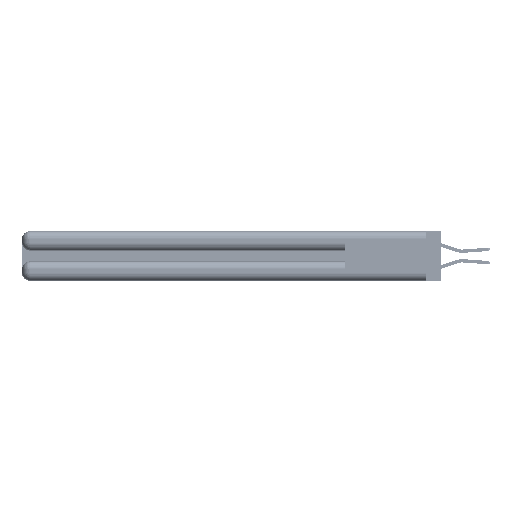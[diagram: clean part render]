
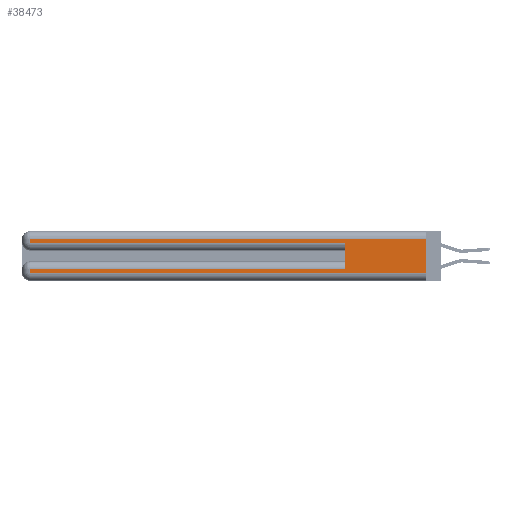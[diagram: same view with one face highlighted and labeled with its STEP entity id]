
A CAD part, left-side view. The second image highlights one B-rep face of the part: STEP entity #38473.
In plain terms, the highlighted planar face has unit normal (-1, 0, 0).
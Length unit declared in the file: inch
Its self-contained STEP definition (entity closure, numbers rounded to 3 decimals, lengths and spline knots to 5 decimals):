
#890 = CARTESIAN_POINT ( 'NONE',  ( 0., 2.94, 0.37 ) ) ;
#932 = VERTEX_POINT ( 'NONE', #32620 ) ;
#1877 = EDGE_CURVE ( 'NONE', #35243, #2897, #27796, .T. ) ;
#2897 = VERTEX_POINT ( 'NONE', #12723 ) ;
#3197 = ORIENTED_EDGE ( 'NONE', *, *, #33823, .F. ) ;
#3371 = CARTESIAN_POINT ( 'NONE',  ( 0., 0.6, 0.285 ) ) ;
#3842 = AXIS2_PLACEMENT_3D ( 'NONE', #46425, #28708, #24818 ) ;
#5562 = LINE ( 'NONE', #17791, #46593 ) ;
#5864 = DIRECTION ( 'NONE',  ( 0., -1., 0. ) ) ;
#5989 = CARTESIAN_POINT ( 'NONE',  ( 0., 2.94, 0.37 ) ) ;
#6622 = CARTESIAN_POINT ( 'NONE',  ( 0., 0., 0.06 ) ) ;
#7328 = DIRECTION ( 'NONE',  ( 0., 0., -1. ) ) ;
#9980 = VECTOR ( 'NONE', #13212, 39.37008 ) ;
#10544 = ORIENTED_EDGE ( 'NONE', *, *, #23265, .T. ) ;
#11126 = VECTOR ( 'NONE', #21945, 39.37008 ) ;
#11257 = ORIENTED_EDGE ( 'NONE', *, *, #32932, .T. ) ;
#11931 = ORIENTED_EDGE ( 'NONE', *, *, #38684, .T. ) ;
#12723 = CARTESIAN_POINT ( 'NONE',  ( 0., 0., 0.06 ) ) ;
#13212 = DIRECTION ( 'NONE',  ( 0., 0., -1. ) ) ;
#14539 = LINE ( 'NONE', #35554, #11126 ) ;
#15674 = VERTEX_POINT ( 'NONE', #33272 ) ;
#16194 = VERTEX_POINT ( 'NONE', #19778 ) ;
#17791 = CARTESIAN_POINT ( 'NONE',  ( 0., 0., 0.285 ) ) ;
#19778 = CARTESIAN_POINT ( 'NONE',  ( 0., 2.94, 0.085 ) ) ;
#20810 = ORIENTED_EDGE ( 'NONE', *, *, #1877, .F. ) ;
#21945 = DIRECTION ( 'NONE',  ( 0., 1., 0. ) ) ;
#21985 = CARTESIAN_POINT ( 'NONE',  ( 0., 0., 0.37 ) ) ;
#23182 = VECTOR ( 'NONE', #54399, 39.37008 ) ;
#23265 = EDGE_CURVE ( 'NONE', #15674, #24931, #47093, .T. ) ;
#23719 = VECTOR ( 'NONE', #32112, 39.37008 ) ;
#24041 = LINE ( 'NONE', #6622, #41199 ) ;
#24818 = DIRECTION ( 'NONE',  ( 0., 0., -1. ) ) ;
#24931 = VERTEX_POINT ( 'NONE', #40287 ) ;
#25296 = EDGE_LOOP ( 'NONE', ( #20810, #11931, #10544, #47785, #3197, #11257, #41874, #27517 ) ) ;
#27302 = DIRECTION ( 'NONE',  ( 0., 0., -1. ) ) ;
#27517 = ORIENTED_EDGE ( 'NONE', *, *, #31143, .T. ) ;
#27543 = EDGE_CURVE ( 'NONE', #16194, #932, #53523, .T. ) ;
#27796 = LINE ( 'NONE', #21985, #9980 ) ;
#28708 = DIRECTION ( 'NONE',  ( 1., 0., 0. ) ) ;
#30741 = LINE ( 'NONE', #32299, #23182 ) ;
#31143 = EDGE_CURVE ( 'NONE', #932, #2897, #24041, .T. ) ;
#32112 = DIRECTION ( 'NONE',  ( 0., 0., 1. ) ) ;
#32299 = CARTESIAN_POINT ( 'NONE',  ( 0., 0., 0.085 ) ) ;
#32620 = CARTESIAN_POINT ( 'NONE',  ( 0., 2.94, 0.06 ) ) ;
#32932 = EDGE_CURVE ( 'NONE', #41342, #16194, #30741, .T. ) ;
#33272 = CARTESIAN_POINT ( 'NONE',  ( 0., 2.94, 0.31 ) ) ;
#33823 = EDGE_CURVE ( 'NONE', #41342, #43719, #39517, .T. ) ;
#34860 = VECTOR ( 'NONE', #27302, 39.37008 ) ;
#35243 = VERTEX_POINT ( 'NONE', #54662 ) ;
#35554 = CARTESIAN_POINT ( 'NONE',  ( 0., 0., 0.31 ) ) ;
#38473 = ADVANCED_FACE ( 'NONE', ( #53553 ), #55399, .F. ) ;
#38684 = EDGE_CURVE ( 'NONE', #35243, #15674, #14539, .T. ) ;
#39517 = LINE ( 'NONE', #49441, #23719 ) ;
#40287 = CARTESIAN_POINT ( 'NONE',  ( 0., 2.94, 0.285 ) ) ;
#41199 = VECTOR ( 'NONE', #5864, 39.37008 ) ;
#41342 = VERTEX_POINT ( 'NONE', #48797 ) ;
#41874 = ORIENTED_EDGE ( 'NONE', *, *, #27543, .T. ) ;
#43719 = VERTEX_POINT ( 'NONE', #3371 ) ;
#46425 = CARTESIAN_POINT ( 'NONE',  ( 0., 0., 0.37 ) ) ;
#46593 = VECTOR ( 'NONE', #52581, 39.37008 ) ;
#46753 = EDGE_CURVE ( 'NONE', #24931, #43719, #5562, .T. ) ;
#47093 = LINE ( 'NONE', #890, #34860 ) ;
#47785 = ORIENTED_EDGE ( 'NONE', *, *, #46753, .T. ) ;
#48043 = VECTOR ( 'NONE', #7328, 39.37008 ) ;
#48797 = CARTESIAN_POINT ( 'NONE',  ( 0., 0.6, 0.085 ) ) ;
#49441 = CARTESIAN_POINT ( 'NONE',  ( 0., 0.6, 0.145 ) ) ;
#52581 = DIRECTION ( 'NONE',  ( 0., -1., 0. ) ) ;
#53523 = LINE ( 'NONE', #5989, #48043 ) ;
#53553 = FACE_OUTER_BOUND ( 'NONE', #25296, .T. ) ;
#54399 = DIRECTION ( 'NONE',  ( 0., 1., 0. ) ) ;
#54662 = CARTESIAN_POINT ( 'NONE',  ( 0., 0., 0.31 ) ) ;
#55399 = PLANE ( 'NONE',  #3842 ) ;
